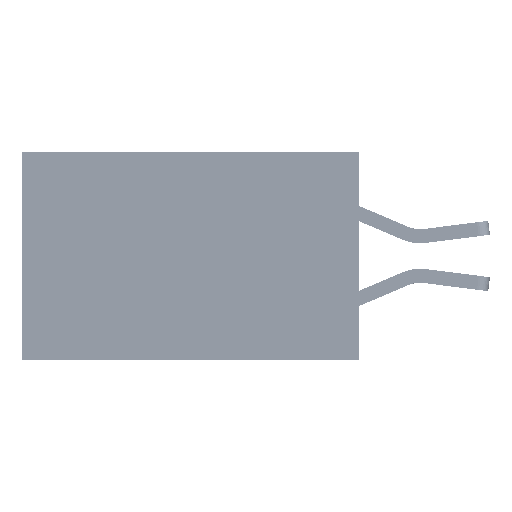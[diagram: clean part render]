
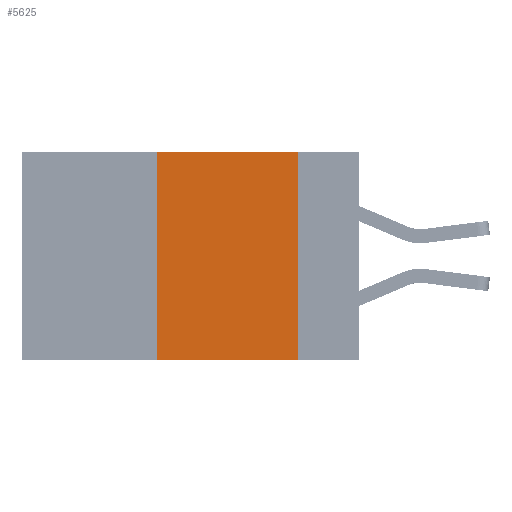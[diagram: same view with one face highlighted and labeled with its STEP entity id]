
A CAD part, left-side view. The second image highlights one B-rep face of the part: STEP entity #5625.
In plain terms, the highlighted planar face has unit normal (-1, 0, 0).
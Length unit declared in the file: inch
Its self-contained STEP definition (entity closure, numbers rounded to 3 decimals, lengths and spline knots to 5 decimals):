
#537 = DIRECTION ( 'NONE',  ( 0., -1., 0. ) ) ;
#2698 = CARTESIAN_POINT ( 'NONE',  ( 0., 0.11, 0. ) ) ;
#4204 = CARTESIAN_POINT ( 'NONE',  ( 0., 0.11, 0. ) ) ;
#5395 = LINE ( 'NONE', #4204, #9552 ) ;
#5625 = ADVANCED_FACE ( 'NONE', ( #10892 ), #29950, .F. ) ;
#6336 = DIRECTION ( 'NONE',  ( 0., 0., -1. ) ) ;
#6518 = CARTESIAN_POINT ( 'NONE',  ( 0., 0.36, 0. ) ) ;
#6844 = EDGE_CURVE ( 'NONE', #24885, #30129, #33520, .T. ) ;
#7179 = EDGE_LOOP ( 'NONE', ( #26580, #21140, #24755, #17524 ) ) ;
#8767 = AXIS2_PLACEMENT_3D ( 'NONE', #21171, #9572, #6336 ) ;
#9279 = VERTEX_POINT ( 'NONE', #22081 ) ;
#9552 = VECTOR ( 'NONE', #31200, 39.37008 ) ;
#9572 = DIRECTION ( 'NONE',  ( 1., 0., 0. ) ) ;
#10892 = FACE_OUTER_BOUND ( 'NONE', #7179, .T. ) ;
#12451 = EDGE_CURVE ( 'NONE', #30129, #32996, #24544, .T. ) ;
#12953 = DIRECTION ( 'NONE',  ( 0., -1., 0. ) ) ;
#13408 = CARTESIAN_POINT ( 'NONE',  ( 0., 0.36, 0. ) ) ;
#13841 = CARTESIAN_POINT ( 'NONE',  ( 0., 0.36, -0.37 ) ) ;
#17524 = ORIENTED_EDGE ( 'NONE', *, *, #28879, .T. ) ;
#20818 = LINE ( 'NONE', #30970, #27802 ) ;
#21140 = ORIENTED_EDGE ( 'NONE', *, *, #12451, .F. ) ;
#21171 = CARTESIAN_POINT ( 'NONE',  ( 0., 0.6, 0. ) ) ;
#22081 = CARTESIAN_POINT ( 'NONE',  ( 0., 0.11, -0.37 ) ) ;
#22667 = VECTOR ( 'NONE', #537, 39.37008 ) ;
#24544 = LINE ( 'NONE', #33455, #22667 ) ;
#24755 = ORIENTED_EDGE ( 'NONE', *, *, #6844, .F. ) ;
#24885 = VERTEX_POINT ( 'NONE', #13841 ) ;
#26580 = ORIENTED_EDGE ( 'NONE', *, *, #29562, .F. ) ;
#27802 = VECTOR ( 'NONE', #12953, 39.37008 ) ;
#28879 = EDGE_CURVE ( 'NONE', #24885, #9279, #20818, .T. ) ;
#29562 = EDGE_CURVE ( 'NONE', #32996, #9279, #5395, .T. ) ;
#29950 = PLANE ( 'NONE',  #8767 ) ;
#30129 = VERTEX_POINT ( 'NONE', #6518 ) ;
#30970 = CARTESIAN_POINT ( 'NONE',  ( 0., 0.6, -0.37 ) ) ;
#31200 = DIRECTION ( 'NONE',  ( 0., 0., -1. ) ) ;
#32996 = VERTEX_POINT ( 'NONE', #2698 ) ;
#33455 = CARTESIAN_POINT ( 'NONE',  ( 0., 0.6, 0. ) ) ;
#33520 = LINE ( 'NONE', #13408, #37671 ) ;
#37671 = VECTOR ( 'NONE', #38019, 39.37008 ) ;
#38019 = DIRECTION ( 'NONE',  ( 0., 0., 1. ) ) ;
